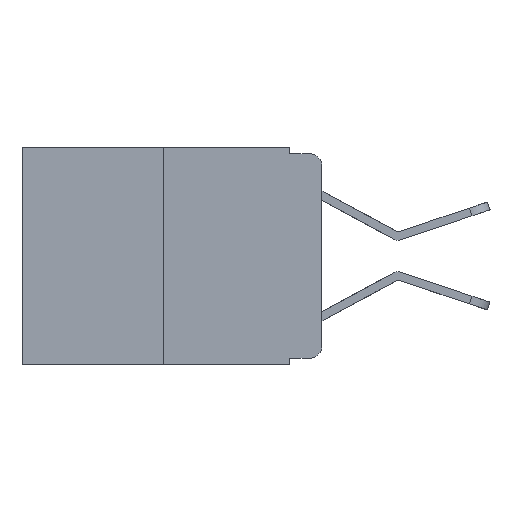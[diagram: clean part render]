
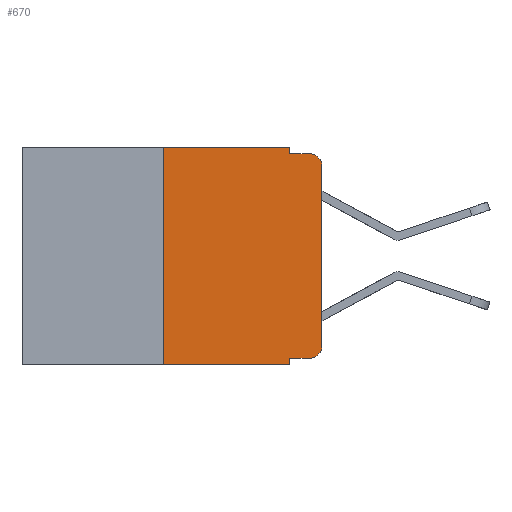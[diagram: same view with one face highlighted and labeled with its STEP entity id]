
A CAD part, left-side view. The second image highlights one B-rep face of the part: STEP entity #670.
In plain terms, the highlighted planar face has unit normal (-1, 0, 0).
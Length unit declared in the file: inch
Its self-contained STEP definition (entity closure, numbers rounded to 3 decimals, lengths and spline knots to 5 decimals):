
#587 = VERTEX_POINT ( 'NONE', #13759 ) ;
#596 = LINE ( 'NONE', #17374, #9699 ) ;
#670 = ADVANCED_FACE ( 'NONE', ( #8578 ), #15236, .F. ) ;
#980 = DIRECTION ( 'NONE',  ( 0., -1., 0. ) ) ;
#1027 = CARTESIAN_POINT ( 'NONE',  ( 0., 0., -0.313 ) ) ;
#1072 = CIRCLE ( 'NONE', #5878, 0.02 ) ;
#1476 = ORIENTED_EDGE ( 'NONE', *, *, #19479, .T. ) ;
#2271 = VECTOR ( 'NONE', #980, 39.37008 ) ;
#2475 = CARTESIAN_POINT ( 'NONE',  ( 0., 0.051, 0. ) ) ;
#2878 = EDGE_CURVE ( 'NONE', #10323, #12611, #8397, .T. ) ;
#2968 = AXIS2_PLACEMENT_3D ( 'NONE', #6230, #18896, #8051 ) ;
#2982 = CARTESIAN_POINT ( 'NONE',  ( 0., 0.25, -0.343 ) ) ;
#3069 = CARTESIAN_POINT ( 'NONE',  ( 0., 0.051, -0.01 ) ) ;
#3167 = ORIENTED_EDGE ( 'NONE', *, *, #20412, .F. ) ;
#3327 = LINE ( 'NONE', #12623, #21957 ) ;
#3406 = DIRECTION ( 'NONE',  ( -1., 0., 0. ) ) ;
#3437 = ORIENTED_EDGE ( 'NONE', *, *, #9171, .T. ) ;
#3457 = ORIENTED_EDGE ( 'NONE', *, *, #17665, .F. ) ;
#3883 = LINE ( 'NONE', #17992, #17771 ) ;
#4270 = LINE ( 'NONE', #15201, #18165 ) ;
#4349 = DIRECTION ( 'NONE',  ( 0., -1., 0. ) ) ;
#4804 = CARTESIAN_POINT ( 'NONE',  ( 0., 0.25, 0. ) ) ;
#4950 = CARTESIAN_POINT ( 'NONE',  ( 0., 0.051, 0. ) ) ;
#5474 = VERTEX_POINT ( 'NONE', #14099 ) ;
#5675 = EDGE_LOOP ( 'NONE', ( #3437, #8834, #15349, #16489, #3167, #13936, #10839, #3457, #19058, #1476 ) ) ;
#5878 = AXIS2_PLACEMENT_3D ( 'NONE', #14256, #3406, #16062 ) ;
#5977 = VERTEX_POINT ( 'NONE', #2982 ) ;
#6230 = CARTESIAN_POINT ( 'NONE',  ( 0., 0.473, 0. ) ) ;
#6535 = DIRECTION ( 'NONE',  ( 0., 0., -1. ) ) ;
#6703 = CARTESIAN_POINT ( 'NONE',  ( 0., 0.051, -0.343 ) ) ;
#7074 = CARTESIAN_POINT ( 'NONE',  ( 0., 0.051, -0.01 ) ) ;
#7263 = DIRECTION ( 'NONE',  ( 0., -1., 0. ) ) ;
#7608 = LINE ( 'NONE', #2475, #16660 ) ;
#7644 = VERTEX_POINT ( 'NONE', #6703 ) ;
#8051 = DIRECTION ( 'NONE',  ( 0., 0., -1. ) ) ;
#8397 = LINE ( 'NONE', #7074, #22189 ) ;
#8578 = FACE_OUTER_BOUND ( 'NONE', #5675, .T. ) ;
#8834 = ORIENTED_EDGE ( 'NONE', *, *, #22152, .T. ) ;
#8982 = VERTEX_POINT ( 'NONE', #4950 ) ;
#9171 = EDGE_CURVE ( 'NONE', #11536, #5474, #17029, .T. ) ;
#9699 = VECTOR ( 'NONE', #6535, 39.37008 ) ;
#9876 = CARTESIAN_POINT ( 'NONE',  ( 0., 0.02, -0.03 ) ) ;
#10323 = VERTEX_POINT ( 'NONE', #3069 ) ;
#10839 = ORIENTED_EDGE ( 'NONE', *, *, #13440, .T. ) ;
#11396 = EDGE_CURVE ( 'NONE', #8982, #10323, #7608, .T. ) ;
#11536 = VERTEX_POINT ( 'NONE', #1027 ) ;
#11705 = DIRECTION ( 'NONE',  ( 0., 0., -1. ) ) ;
#11777 = EDGE_CURVE ( 'NONE', #5977, #21695, #3883, .T. ) ;
#11915 = LINE ( 'NONE', #15481, #2271 ) ;
#12611 = VERTEX_POINT ( 'NONE', #19393 ) ;
#12623 = CARTESIAN_POINT ( 'NONE',  ( 0., 0.473, -0.343 ) ) ;
#13058 = AXIS2_PLACEMENT_3D ( 'NONE', #9876, #22432, #11705 ) ;
#13440 = EDGE_CURVE ( 'NONE', #5977, #7644, #3327, .T. ) ;
#13759 = CARTESIAN_POINT ( 'NONE',  ( 0., 0.02, -0.333 ) ) ;
#13936 = ORIENTED_EDGE ( 'NONE', *, *, #11777, .F. ) ;
#14099 = CARTESIAN_POINT ( 'NONE',  ( 0., 0., -0.03 ) ) ;
#14256 = CARTESIAN_POINT ( 'NONE',  ( 0., 0.02, -0.313 ) ) ;
#15145 = DIRECTION ( 'NONE',  ( 0., 0., -1. ) ) ;
#15201 = CARTESIAN_POINT ( 'NONE',  ( 0., 0.051, -0.333 ) ) ;
#15236 = PLANE ( 'NONE',  #2968 ) ;
#15349 = ORIENTED_EDGE ( 'NONE', *, *, #2878, .F. ) ;
#15481 = CARTESIAN_POINT ( 'NONE',  ( 0., 0.473, 0. ) ) ;
#16062 = DIRECTION ( 'NONE',  ( 0., 0., -1. ) ) ;
#16393 = CIRCLE ( 'NONE', #13058, 0.02 ) ;
#16489 = ORIENTED_EDGE ( 'NONE', *, *, #11396, .F. ) ;
#16660 = VECTOR ( 'NONE', #15145, 39.37008 ) ;
#16970 = CARTESIAN_POINT ( 'NONE',  ( 0., 0.051, -0.333 ) ) ;
#17029 = LINE ( 'NONE', #18097, #20666 ) ;
#17374 = CARTESIAN_POINT ( 'NONE',  ( 0., 0.051, 0. ) ) ;
#17665 = EDGE_CURVE ( 'NONE', #19176, #7644, #596, .T. ) ;
#17771 = VECTOR ( 'NONE', #21487, 39.37008 ) ;
#17992 = CARTESIAN_POINT ( 'NONE',  ( 0., 0.25, 0. ) ) ;
#18097 = CARTESIAN_POINT ( 'NONE',  ( 0., 0., 0. ) ) ;
#18165 = VECTOR ( 'NONE', #4349, 39.37008 ) ;
#18222 = EDGE_CURVE ( 'NONE', #19176, #587, #4270, .T. ) ;
#18896 = DIRECTION ( 'NONE',  ( 1., 0., 0. ) ) ;
#19058 = ORIENTED_EDGE ( 'NONE', *, *, #18222, .T. ) ;
#19176 = VERTEX_POINT ( 'NONE', #16970 ) ;
#19393 = CARTESIAN_POINT ( 'NONE',  ( 0., 0.02, -0.01 ) ) ;
#19479 = EDGE_CURVE ( 'NONE', #587, #11536, #1072, .T. ) ;
#20412 = EDGE_CURVE ( 'NONE', #21695, #8982, #11915, .T. ) ;
#20666 = VECTOR ( 'NONE', #21670, 39.37008 ) ;
#21487 = DIRECTION ( 'NONE',  ( 0., 0., 1. ) ) ;
#21493 = DIRECTION ( 'NONE',  ( 0., -1., 0. ) ) ;
#21670 = DIRECTION ( 'NONE',  ( 0., 0., 1. ) ) ;
#21695 = VERTEX_POINT ( 'NONE', #4804 ) ;
#21957 = VECTOR ( 'NONE', #7263, 39.37008 ) ;
#22152 = EDGE_CURVE ( 'NONE', #5474, #12611, #16393, .T. ) ;
#22189 = VECTOR ( 'NONE', #21493, 39.37008 ) ;
#22432 = DIRECTION ( 'NONE',  ( -1., 0., 0. ) ) ;
